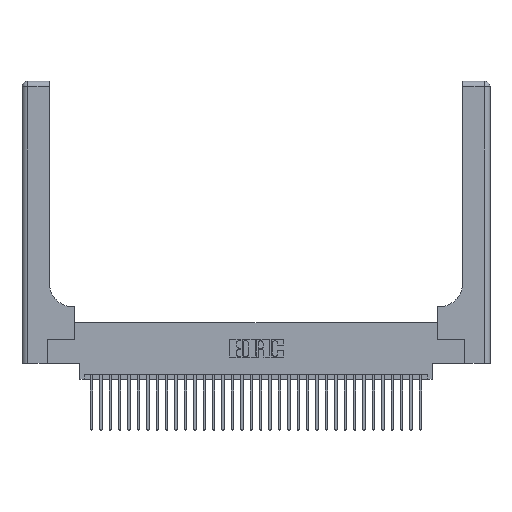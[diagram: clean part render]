
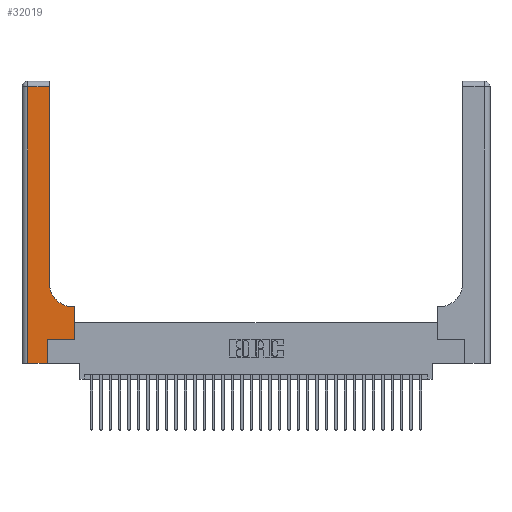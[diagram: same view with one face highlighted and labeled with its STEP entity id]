
A CAD part, top view. The second image highlights one B-rep face of the part: STEP entity #32019.
In plain terms, the highlighted planar face has unit normal (0, 0, 1).
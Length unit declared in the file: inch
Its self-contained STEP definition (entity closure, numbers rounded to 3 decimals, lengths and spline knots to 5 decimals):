
#47 = CARTESIAN_POINT ( 'NONE',  ( 0.06, 3., 0.37 ) ) ;
#630 = CARTESIAN_POINT ( 'NONE',  ( 0.269, 0.25, 0.37 ) ) ;
#915 = DIRECTION ( 'NONE',  ( 1., 0., 0. ) ) ;
#932 = ORIENTED_EDGE ( 'NONE', *, *, #15214, .T. ) ;
#1033 = CARTESIAN_POINT ( 'NONE',  ( 0.2915, 2.94, 0.37 ) ) ;
#1727 = CARTESIAN_POINT ( 'NONE',  ( 0.06, 0., 0.37 ) ) ;
#2093 = EDGE_CURVE ( 'NONE', #26131, #33697, #26617, .T. ) ;
#2289 = EDGE_CURVE ( 'NONE', #32665, #11715, #7563, .T. ) ;
#2670 = ORIENTED_EDGE ( 'NONE', *, *, #17687, .T. ) ;
#3561 = VECTOR ( 'NONE', #11005, 39.37008 ) ;
#5278 = CARTESIAN_POINT ( 'NONE',  ( 0., 2.94, 0.37 ) ) ;
#5388 = DIRECTION ( 'NONE',  ( -1., 0., 0. ) ) ;
#5441 = CARTESIAN_POINT ( 'NONE',  ( 0.269, 0.25, 0.37 ) ) ;
#6117 = CIRCLE ( 'NONE', #12277, 0.25 ) ;
#7094 = LINE ( 'NONE', #5278, #27394 ) ;
#7563 = LINE ( 'NONE', #31773, #23751 ) ;
#8565 = ORIENTED_EDGE ( 'NONE', *, *, #11409, .T. ) ;
#9045 = DIRECTION ( 'NONE',  ( 0., 1., 0. ) ) ;
#9095 = VECTOR ( 'NONE', #29086, 39.37008 ) ;
#9409 = CARTESIAN_POINT ( 'NONE',  ( 0.5585, 0.25, 0.37 ) ) ;
#9685 = VERTEX_POINT ( 'NONE', #1727 ) ;
#9811 = VECTOR ( 'NONE', #31213, 39.37008 ) ;
#9853 = LINE ( 'NONE', #5441, #3561 ) ;
#9890 = DIRECTION ( 'NONE',  ( 1., 0., 0. ) ) ;
#9943 = ORIENTED_EDGE ( 'NONE', *, *, #24280, .T. ) ;
#10098 = CARTESIAN_POINT ( 'NONE',  ( 0.269, 0., 0.37 ) ) ;
#11005 = DIRECTION ( 'NONE',  ( 1., 0., 0. ) ) ;
#11223 = ORIENTED_EDGE ( 'NONE', *, *, #2289, .T. ) ;
#11409 = EDGE_CURVE ( 'NONE', #33697, #32665, #6117, .T. ) ;
#11519 = CARTESIAN_POINT ( 'NONE',  ( 0.5415, 0.85, 0.37 ) ) ;
#11715 = VERTEX_POINT ( 'NONE', #1033 ) ;
#12277 = AXIS2_PLACEMENT_3D ( 'NONE', #11519, #30077, #915 ) ;
#13851 = VECTOR ( 'NONE', #9890, 39.37008 ) ;
#14452 = ORIENTED_EDGE ( 'NONE', *, *, #14565, .T. ) ;
#14453 = CARTESIAN_POINT ( 'NONE',  ( 0.06, 2.94, 0.37 ) ) ;
#14565 = EDGE_CURVE ( 'NONE', #28460, #26131, #27357, .T. ) ;
#15214 = EDGE_CURVE ( 'NONE', #11715, #15710, #7094, .T. ) ;
#15225 = CARTESIAN_POINT ( 'NONE',  ( 0.5415, 0.6, 0.37 ) ) ;
#15710 = VERTEX_POINT ( 'NONE', #14453 ) ;
#15911 = DIRECTION ( 'NONE',  ( 0., 1., 0. ) ) ;
#16530 = VERTEX_POINT ( 'NONE', #18109 ) ;
#16906 = DIRECTION ( 'NONE',  ( -1., 0., 0. ) ) ;
#17687 = EDGE_CURVE ( 'NONE', #16530, #18982, #28480, .T. ) ;
#17882 = LINE ( 'NONE', #47, #9095 ) ;
#17918 = CARTESIAN_POINT ( 'NONE',  ( 0.5585, 0.6, 0.37 ) ) ;
#18109 = CARTESIAN_POINT ( 'NONE',  ( 0.269, 0., 0.37 ) ) ;
#18428 = EDGE_LOOP ( 'NONE', ( #11223, #932, #23705, #23400, #2670, #9943, #14452, #30845, #8565 ) ) ;
#18982 = VERTEX_POINT ( 'NONE', #630 ) ;
#19780 = DIRECTION ( 'NONE',  ( -1., 0., 0. ) ) ;
#21466 = AXIS2_PLACEMENT_3D ( 'NONE', #29994, #30228, #19780 ) ;
#23400 = ORIENTED_EDGE ( 'NONE', *, *, #31464, .T. ) ;
#23705 = ORIENTED_EDGE ( 'NONE', *, *, #33897, .T. ) ;
#23751 = VECTOR ( 'NONE', #15911, 39.37008 ) ;
#24280 = EDGE_CURVE ( 'NONE', #18982, #28460, #9853, .T. ) ;
#25403 = VECTOR ( 'NONE', #16906, 39.37008 ) ;
#26131 = VERTEX_POINT ( 'NONE', #17918 ) ;
#26617 = LINE ( 'NONE', #30566, #25403 ) ;
#27085 = FACE_OUTER_BOUND ( 'NONE', #18428, .T. ) ;
#27357 = LINE ( 'NONE', #9409, #31586 ) ;
#27394 = VECTOR ( 'NONE', #5388, 39.37008 ) ;
#27561 = PLANE ( 'NONE',  #21466 ) ;
#27606 = CARTESIAN_POINT ( 'NONE',  ( 0., 0., 0.37 ) ) ;
#27886 = CARTESIAN_POINT ( 'NONE',  ( 0.2915, 0.85, 0.37 ) ) ;
#27957 = LINE ( 'NONE', #27606, #13851 ) ;
#28460 = VERTEX_POINT ( 'NONE', #31123 ) ;
#28480 = LINE ( 'NONE', #10098, #9811 ) ;
#29086 = DIRECTION ( 'NONE',  ( 0., -1., 0. ) ) ;
#29994 = CARTESIAN_POINT ( 'NONE',  ( 0., 3., 0.37 ) ) ;
#30077 = DIRECTION ( 'NONE',  ( 0., 0., -1. ) ) ;
#30228 = DIRECTION ( 'NONE',  ( 0., 0., -1. ) ) ;
#30566 = CARTESIAN_POINT ( 'NONE',  ( 0.2915, 0.6, 0.37 ) ) ;
#30845 = ORIENTED_EDGE ( 'NONE', *, *, #2093, .T. ) ;
#31123 = CARTESIAN_POINT ( 'NONE',  ( 0.5585, 0.25, 0.37 ) ) ;
#31213 = DIRECTION ( 'NONE',  ( 0., 1., 0. ) ) ;
#31464 = EDGE_CURVE ( 'NONE', #9685, #16530, #27957, .T. ) ;
#31586 = VECTOR ( 'NONE', #9045, 39.37008 ) ;
#31773 = CARTESIAN_POINT ( 'NONE',  ( 0.2915, 3., 0.37 ) ) ;
#32019 = ADVANCED_FACE ( 'NONE', ( #27085 ), #27561, .F. ) ;
#32665 = VERTEX_POINT ( 'NONE', #27886 ) ;
#33697 = VERTEX_POINT ( 'NONE', #15225 ) ;
#33897 = EDGE_CURVE ( 'NONE', #15710, #9685, #17882, .T. ) ;
